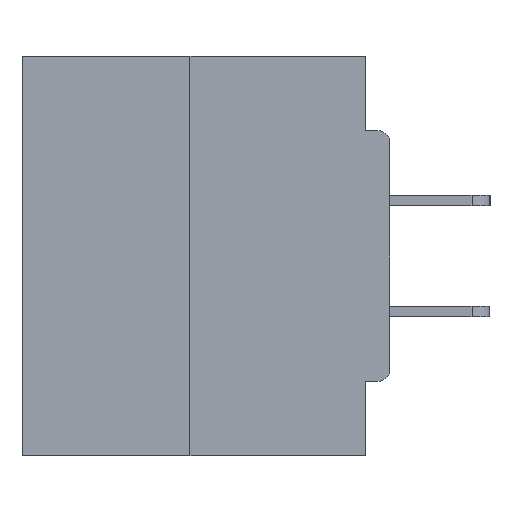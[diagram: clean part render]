
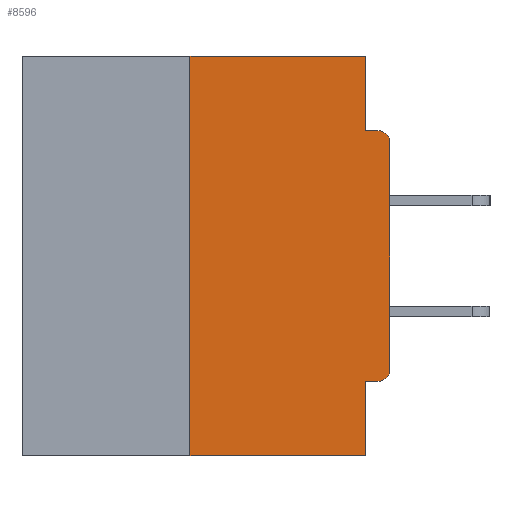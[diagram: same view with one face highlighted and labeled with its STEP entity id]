
A CAD part, left-side view. The second image highlights one B-rep face of the part: STEP entity #8596.
In plain terms, the highlighted planar face has unit normal (-1, 0, 0).
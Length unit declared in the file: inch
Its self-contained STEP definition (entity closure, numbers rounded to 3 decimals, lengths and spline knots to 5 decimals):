
#273 = VERTEX_POINT ( 'NONE', #2044 ) ;
#620 = EDGE_CURVE ( 'NONE', #7696, #5846, #7134, .T. ) ;
#1205 = EDGE_CURVE ( 'NONE', #5846, #16836, #26881, .T. ) ;
#1229 = DIRECTION ( 'NONE',  ( 0., -1., 0. ) ) ;
#1266 = LINE ( 'NONE', #17808, #25426 ) ;
#1574 = AXIS2_PLACEMENT_3D ( 'NONE', #18729, #13750, #27601 ) ;
#1843 = VECTOR ( 'NONE', #1229, 39.37008 ) ;
#1893 = CARTESIAN_POINT ( 'NONE',  ( 0., 0.015, -0.3915 ) ) ;
#2044 = CARTESIAN_POINT ( 'NONE',  ( 0., 0.031, -0.5 ) ) ;
#2423 = DIRECTION ( 'NONE',  ( 0., 0., -1. ) ) ;
#2940 = EDGE_CURVE ( 'NONE', #12957, #14700, #18822, .T. ) ;
#3093 = ORIENTED_EDGE ( 'NONE', *, *, #3943, .F. ) ;
#3404 = VECTOR ( 'NONE', #16861, 39.37008 ) ;
#3916 = CARTESIAN_POINT ( 'NONE',  ( 0., 0., -0.0935 ) ) ;
#3943 = EDGE_CURVE ( 'NONE', #7696, #26886, #17935, .T. ) ;
#4222 = DIRECTION ( 'NONE',  ( 0., 0., -1. ) ) ;
#4719 = CARTESIAN_POINT ( 'NONE',  ( 0., 0.25, 0. ) ) ;
#4737 = CARTESIAN_POINT ( 'NONE',  ( 0., 0.031, -0.4065 ) ) ;
#4884 = CARTESIAN_POINT ( 'NONE',  ( 0., 0.25, -0.5 ) ) ;
#5066 = EDGE_CURVE ( 'NONE', #26886, #273, #13436, .T. ) ;
#5392 = DIRECTION ( 'NONE',  ( 0., 1., 0. ) ) ;
#5573 = AXIS2_PLACEMENT_3D ( 'NONE', #17540, #27992, #2423 ) ;
#5846 = VERTEX_POINT ( 'NONE', #16894 ) ;
#6365 = VECTOR ( 'NONE', #13426, 39.37008 ) ;
#7134 = CIRCLE ( 'NONE', #17720, 0.015 ) ;
#7696 = VERTEX_POINT ( 'NONE', #15009 ) ;
#7947 = CARTESIAN_POINT ( 'NONE',  ( 0., 0., -0.1085 ) ) ;
#8445 = CARTESIAN_POINT ( 'NONE',  ( 0., 0.015, -0.0935 ) ) ;
#8596 = ADVANCED_FACE ( 'NONE', ( #14411 ), #23730, .F. ) ;
#9641 = ORIENTED_EDGE ( 'NONE', *, *, #14967, .F. ) ;
#10220 = CARTESIAN_POINT ( 'NONE',  ( 0., 0., 0. ) ) ;
#10336 = CARTESIAN_POINT ( 'NONE',  ( 0., 0.25, 0. ) ) ;
#10494 = CIRCLE ( 'NONE', #5573, 0.015 ) ;
#11295 = ORIENTED_EDGE ( 'NONE', *, *, #620, .T. ) ;
#12414 = VECTOR ( 'NONE', #13784, 39.37008 ) ;
#12816 = DIRECTION ( 'NONE',  ( 0., -1., 0. ) ) ;
#12957 = VERTEX_POINT ( 'NONE', #4884 ) ;
#13313 = CARTESIAN_POINT ( 'NONE',  ( 0., 0.031, -0.0935 ) ) ;
#13343 = DIRECTION ( 'NONE',  ( 0., -1., 0. ) ) ;
#13426 = DIRECTION ( 'NONE',  ( 0., 0., -1. ) ) ;
#13436 = LINE ( 'NONE', #30853, #6365 ) ;
#13750 = DIRECTION ( 'NONE',  ( 1., 0., 0. ) ) ;
#13784 = DIRECTION ( 'NONE',  ( 0., 0., -1. ) ) ;
#14157 = LINE ( 'NONE', #3916, #1843 ) ;
#14411 = FACE_OUTER_BOUND ( 'NONE', #18931, .T. ) ;
#14700 = VERTEX_POINT ( 'NONE', #10336 ) ;
#14967 = EDGE_CURVE ( 'NONE', #24175, #23041, #14157, .T. ) ;
#15009 = CARTESIAN_POINT ( 'NONE',  ( 0., 0.015, -0.4065 ) ) ;
#15417 = CARTESIAN_POINT ( 'NONE',  ( 0., 0., -0.4065 ) ) ;
#16273 = EDGE_CURVE ( 'NONE', #16836, #23041, #10494, .T. ) ;
#16382 = ORIENTED_EDGE ( 'NONE', *, *, #1205, .T. ) ;
#16475 = EDGE_CURVE ( 'NONE', #14700, #18461, #27917, .T. ) ;
#16569 = ORIENTED_EDGE ( 'NONE', *, *, #5066, .F. ) ;
#16836 = VERTEX_POINT ( 'NONE', #7947 ) ;
#16861 = DIRECTION ( 'NONE',  ( 0., 0., 1. ) ) ;
#16894 = CARTESIAN_POINT ( 'NONE',  ( 0., 0., -0.3915 ) ) ;
#17012 = DIRECTION ( 'NONE',  ( -1., 0., 0. ) ) ;
#17380 = DIRECTION ( 'NONE',  ( 0., 0., 1. ) ) ;
#17540 = CARTESIAN_POINT ( 'NONE',  ( 0., 0.015, -0.1085 ) ) ;
#17720 = AXIS2_PLACEMENT_3D ( 'NONE', #1893, #17012, #4222 ) ;
#17808 = CARTESIAN_POINT ( 'NONE',  ( 0., 0.46, -0.5 ) ) ;
#17923 = CARTESIAN_POINT ( 'NONE',  ( 0., 0.031, 0. ) ) ;
#17935 = LINE ( 'NONE', #15417, #22692 ) ;
#18461 = VERTEX_POINT ( 'NONE', #17923 ) ;
#18729 = CARTESIAN_POINT ( 'NONE',  ( 0., 0.46, 0. ) ) ;
#18822 = LINE ( 'NONE', #4719, #3404 ) ;
#18931 = EDGE_LOOP ( 'NONE', ( #30677, #21133, #29859, #16569, #3093, #11295, #16382, #26345, #9641, #25262 ) ) ;
#19947 = LINE ( 'NONE', #21204, #12414 ) ;
#20379 = EDGE_CURVE ( 'NONE', #18461, #24175, #19947, .T. ) ;
#21133 = ORIENTED_EDGE ( 'NONE', *, *, #2940, .F. ) ;
#21204 = CARTESIAN_POINT ( 'NONE',  ( 0., 0.031, 0. ) ) ;
#22350 = VECTOR ( 'NONE', #13343, 39.37008 ) ;
#22692 = VECTOR ( 'NONE', #5392, 39.37008 ) ;
#23041 = VERTEX_POINT ( 'NONE', #8445 ) ;
#23730 = PLANE ( 'NONE',  #1574 ) ;
#24175 = VERTEX_POINT ( 'NONE', #13313 ) ;
#25262 = ORIENTED_EDGE ( 'NONE', *, *, #20379, .F. ) ;
#25426 = VECTOR ( 'NONE', #12816, 39.37008 ) ;
#26095 = VECTOR ( 'NONE', #17380, 39.37008 ) ;
#26345 = ORIENTED_EDGE ( 'NONE', *, *, #16273, .T. ) ;
#26881 = LINE ( 'NONE', #10220, #26095 ) ;
#26886 = VERTEX_POINT ( 'NONE', #4737 ) ;
#27601 = DIRECTION ( 'NONE',  ( 0., 0., -1. ) ) ;
#27917 = LINE ( 'NONE', #28544, #22350 ) ;
#27992 = DIRECTION ( 'NONE',  ( -1., 0., 0. ) ) ;
#28544 = CARTESIAN_POINT ( 'NONE',  ( 0., 0.46, 0. ) ) ;
#29178 = EDGE_CURVE ( 'NONE', #12957, #273, #1266, .T. ) ;
#29859 = ORIENTED_EDGE ( 'NONE', *, *, #29178, .T. ) ;
#30677 = ORIENTED_EDGE ( 'NONE', *, *, #16475, .F. ) ;
#30853 = CARTESIAN_POINT ( 'NONE',  ( 0., 0.031, -0.5 ) ) ;
